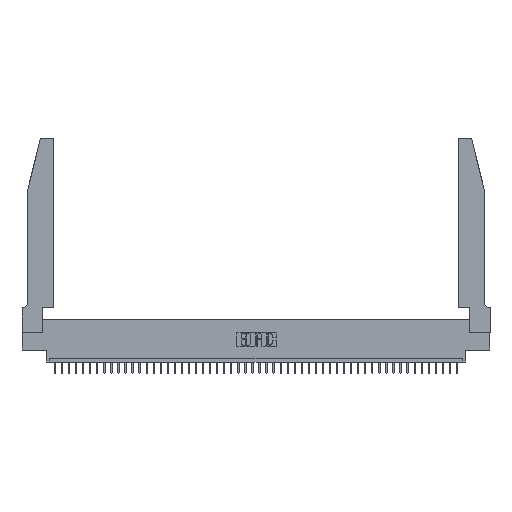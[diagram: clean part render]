
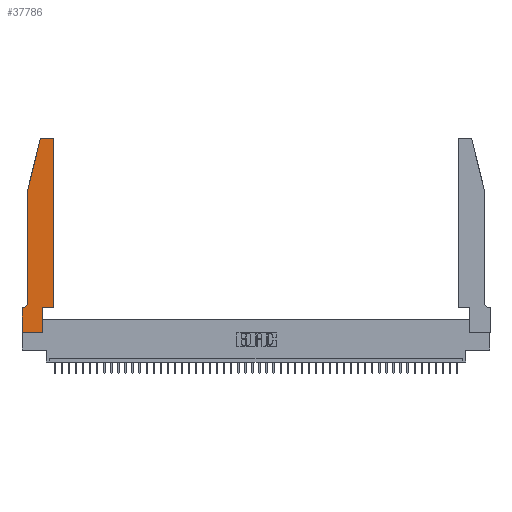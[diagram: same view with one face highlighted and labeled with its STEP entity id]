
A CAD part, top view. The second image highlights one B-rep face of the part: STEP entity #37786.
In plain terms, the highlighted planar face has unit normal (0, 0, 1).
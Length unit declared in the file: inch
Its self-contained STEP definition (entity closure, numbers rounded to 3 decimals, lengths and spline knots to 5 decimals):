
#213 = CARTESIAN_POINT ( 'NONE',  ( 0.2865, 0.35, 0.37 ) ) ;
#286 = ORIENTED_EDGE ( 'NONE', *, *, #32271, .T. ) ;
#964 = EDGE_CURVE ( 'NONE', #45010, #20596, #43924, .T. ) ;
#981 = ORIENTED_EDGE ( 'NONE', *, *, #40552, .T. ) ;
#1158 = VERTEX_POINT ( 'NONE', #14637 ) ;
#1865 = DIRECTION ( 'NONE',  ( -1., 0., 0. ) ) ;
#2302 = CARTESIAN_POINT ( 'NONE',  ( 0.2605, 2.75, 0.37 ) ) ;
#3187 = VECTOR ( 'NONE', #18221, 39.37008 ) ;
#3203 = ORIENTED_EDGE ( 'NONE', *, *, #41015, .T. ) ;
#3240 = VERTEX_POINT ( 'NONE', #10622 ) ;
#3248 = ORIENTED_EDGE ( 'NONE', *, *, #7025, .T. ) ;
#3601 = VECTOR ( 'NONE', #35868, 39.37008 ) ;
#3942 = ORIENTED_EDGE ( 'NONE', *, *, #9581, .T. ) ;
#4236 = VERTEX_POINT ( 'NONE', #20379 ) ;
#4482 = DIRECTION ( 'NONE',  ( 1., 0., 0. ) ) ;
#4486 = CARTESIAN_POINT ( 'NONE',  ( 0.284, 2.72, 0.37 ) ) ;
#4643 = EDGE_CURVE ( 'NONE', #3240, #24337, #41367, .T. ) ;
#4798 = DIRECTION ( 'NONE',  ( 1., 0., 0. ) ) ;
#5188 = VECTOR ( 'NONE', #12906, 39.37008 ) ;
#6844 = ORIENTED_EDGE ( 'NONE', *, *, #26977, .T. ) ;
#6854 = CARTESIAN_POINT ( 'NONE',  ( 0.4205, 2.72, 0.37 ) ) ;
#7013 = CIRCLE ( 'NONE', #24624, 0.07 ) ;
#7025 = EDGE_CURVE ( 'NONE', #18537, #28562, #25452, .T. ) ;
#7183 = LINE ( 'NONE', #44290, #22901 ) ;
#7929 = ORIENTED_EDGE ( 'NONE', *, *, #36166, .T. ) ;
#9475 = LINE ( 'NONE', #23266, #20716 ) ;
#9581 = EDGE_CURVE ( 'NONE', #28562, #3240, #9475, .T. ) ;
#10386 = AXIS2_PLACEMENT_3D ( 'NONE', #6854, #46388, #10578 ) ;
#10496 = VERTEX_POINT ( 'NONE', #11378 ) ;
#10578 = DIRECTION ( 'NONE',  ( 1., 0., 0. ) ) ;
#10622 = CARTESIAN_POINT ( 'NONE',  ( 0.0755, 2., 0.37 ) ) ;
#11378 = CARTESIAN_POINT ( 'NONE',  ( 0.4505, 2.72, 0.37 ) ) ;
#11406 = CARTESIAN_POINT ( 'NONE',  ( 0.0755, 2., 0.37 ) ) ;
#12128 = PLANE ( 'NONE',  #12638 ) ;
#12638 = AXIS2_PLACEMENT_3D ( 'NONE', #26480, #26153, #19407 ) ;
#12906 = DIRECTION ( 'NONE',  ( -1., 0., 0. ) ) ;
#13490 = EDGE_LOOP ( 'NONE', ( #3203, #3248, #3942, #41703, #18242, #34841, #6844, #7929, #981, #25711, #45821, #286 ) ) ;
#13591 = CARTESIAN_POINT ( 'NONE',  ( 0., 0., 0.37 ) ) ;
#13809 = EDGE_CURVE ( 'NONE', #20596, #10496, #7183, .T. ) ;
#14222 = CARTESIAN_POINT ( 'NONE',  ( 0.25487, 2.72718, 0.37 ) ) ;
#14637 = CARTESIAN_POINT ( 'NONE',  ( 0., 0., 0.37 ) ) ;
#15155 = VECTOR ( 'NONE', #1865, 39.37008 ) ;
#15159 = CARTESIAN_POINT ( 'NONE',  ( 0.0755, 0.35, 0.37 ) ) ;
#16933 = VECTOR ( 'NONE', #45952, 39.37008 ) ;
#18221 = DIRECTION ( 'NONE',  ( 0., -1., 0. ) ) ;
#18242 = ORIENTED_EDGE ( 'NONE', *, *, #39985, .T. ) ;
#18427 = VERTEX_POINT ( 'NONE', #19677 ) ;
#18537 = VERTEX_POINT ( 'NONE', #40063 ) ;
#18971 = DIRECTION ( 'NONE',  ( 0., -1., 0. ) ) ;
#19236 = VECTOR ( 'NONE', #4798, 39.37008 ) ;
#19389 = CARTESIAN_POINT ( 'NONE',  ( 0.4505, 0.35, 0.37 ) ) ;
#19407 = DIRECTION ( 'NONE',  ( 1., 0., 0. ) ) ;
#19677 = CARTESIAN_POINT ( 'NONE',  ( 0.0055, 0.35, 0.37 ) ) ;
#20379 = CARTESIAN_POINT ( 'NONE',  ( 0.4205, 2.75, 0.37 ) ) ;
#20596 = VERTEX_POINT ( 'NONE', #19389 ) ;
#20716 = VECTOR ( 'NONE', #21104, 39.37008 ) ;
#21104 = DIRECTION ( 'NONE',  ( -0.239, -0.971, 0. ) ) ;
#22195 = CARTESIAN_POINT ( 'NONE',  ( 0.0055, 0.42, 0.37 ) ) ;
#22901 = VECTOR ( 'NONE', #33655, 39.37008 ) ;
#23266 = CARTESIAN_POINT ( 'NONE',  ( 0.0755, 2., 0.37 ) ) ;
#24337 = VERTEX_POINT ( 'NONE', #38808 ) ;
#24624 = AXIS2_PLACEMENT_3D ( 'NONE', #22195, #29592, #32906 ) ;
#24977 = LINE ( 'NONE', #36158, #3601 ) ;
#25452 = CIRCLE ( 'NONE', #42638, 0.03 ) ;
#25711 = ORIENTED_EDGE ( 'NONE', *, *, #964, .T. ) ;
#25964 = CARTESIAN_POINT ( 'NONE',  ( 0.2865, 0., 0.37 ) ) ;
#26153 = DIRECTION ( 'NONE',  ( 0., 0., 1. ) ) ;
#26307 = CARTESIAN_POINT ( 'NONE',  ( 0.4505, 0.35, 0.37 ) ) ;
#26480 = CARTESIAN_POINT ( 'NONE',  ( 0., 0.35, 0.37 ) ) ;
#26567 = LINE ( 'NONE', #2302, #5188 ) ;
#26746 = LINE ( 'NONE', #40798, #42419 ) ;
#26929 = DIRECTION ( 'NONE',  ( 0., 0., 1. ) ) ;
#26977 = EDGE_CURVE ( 'NONE', #30574, #1158, #26746, .T. ) ;
#28562 = VERTEX_POINT ( 'NONE', #14222 ) ;
#29437 = CIRCLE ( 'NONE', #10386, 0.03 ) ;
#29592 = DIRECTION ( 'NONE',  ( 0., 0., -1. ) ) ;
#30574 = VERTEX_POINT ( 'NONE', #41553 ) ;
#32271 = EDGE_CURVE ( 'NONE', #10496, #4236, #29437, .T. ) ;
#32688 = VERTEX_POINT ( 'NONE', #25964 ) ;
#32906 = DIRECTION ( 'NONE',  ( -1., 0., 0. ) ) ;
#33655 = DIRECTION ( 'NONE',  ( 0., 1., 0. ) ) ;
#34841 = ORIENTED_EDGE ( 'NONE', *, *, #36660, .T. ) ;
#35868 = DIRECTION ( 'NONE',  ( 0., 1., 0. ) ) ;
#36158 = CARTESIAN_POINT ( 'NONE',  ( 0.2865, 0.35, 0.37 ) ) ;
#36166 = EDGE_CURVE ( 'NONE', #1158, #32688, #45560, .T. ) ;
#36660 = EDGE_CURVE ( 'NONE', #18427, #30574, #43791, .T. ) ;
#37786 = ADVANCED_FACE ( 'NONE', ( #45380 ), #12128, .T. ) ;
#38808 = CARTESIAN_POINT ( 'NONE',  ( 0.0755, 0.42, 0.37 ) ) ;
#39985 = EDGE_CURVE ( 'NONE', #24337, #18427, #7013, .T. ) ;
#40063 = CARTESIAN_POINT ( 'NONE',  ( 0.284, 2.75, 0.37 ) ) ;
#40552 = EDGE_CURVE ( 'NONE', #32688, #45010, #24977, .T. ) ;
#40798 = CARTESIAN_POINT ( 'NONE',  ( 0., 0., 0.37 ) ) ;
#41015 = EDGE_CURVE ( 'NONE', #4236, #18537, #26567, .T. ) ;
#41367 = LINE ( 'NONE', #11406, #3187 ) ;
#41553 = CARTESIAN_POINT ( 'NONE',  ( 0., 0.35, 0.37 ) ) ;
#41703 = ORIENTED_EDGE ( 'NONE', *, *, #4643, .T. ) ;
#42419 = VECTOR ( 'NONE', #18971, 39.37008 ) ;
#42638 = AXIS2_PLACEMENT_3D ( 'NONE', #4486, #26929, #4482 ) ;
#43791 = LINE ( 'NONE', #15159, #15155 ) ;
#43924 = LINE ( 'NONE', #26307, #19236 ) ;
#44290 = CARTESIAN_POINT ( 'NONE',  ( 0.4505, 0.35, 0.37 ) ) ;
#45010 = VERTEX_POINT ( 'NONE', #213 ) ;
#45380 = FACE_OUTER_BOUND ( 'NONE', #13490, .T. ) ;
#45560 = LINE ( 'NONE', #13591, #16933 ) ;
#45821 = ORIENTED_EDGE ( 'NONE', *, *, #13809, .T. ) ;
#45952 = DIRECTION ( 'NONE',  ( 1., 0., 0. ) ) ;
#46388 = DIRECTION ( 'NONE',  ( 0., 0., 1. ) ) ;
